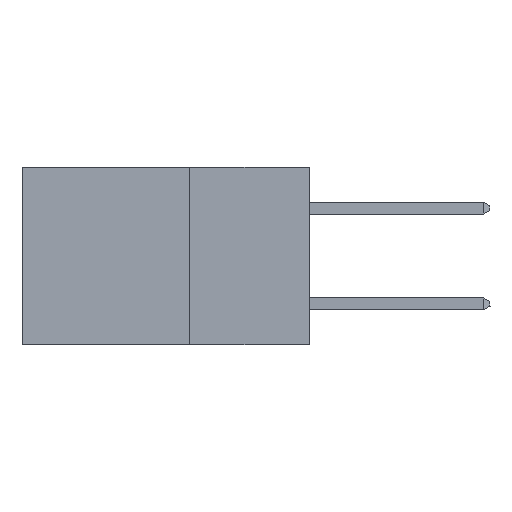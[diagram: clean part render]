
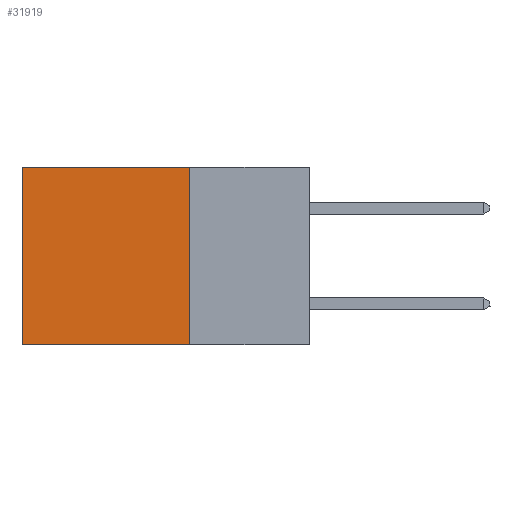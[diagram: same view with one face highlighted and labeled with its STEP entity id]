
A CAD part, left-side view. The second image highlights one B-rep face of the part: STEP entity #31919.
In plain terms, the highlighted planar face has unit normal (-1, 0, 0).
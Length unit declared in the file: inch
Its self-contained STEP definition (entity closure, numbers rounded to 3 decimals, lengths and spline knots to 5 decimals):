
#1154 = VERTEX_POINT ( 'NONE', #10746 ) ;
#1230 = FACE_OUTER_BOUND ( 'NONE', #19401, .T. ) ;
#2661 = PLANE ( 'NONE',  #15347 ) ;
#3942 = DIRECTION ( 'NONE',  ( 0., 0., -1. ) ) ;
#3960 = CARTESIAN_POINT ( 'NONE',  ( 0.2875, 0.25, 0. ) ) ;
#4071 = DIRECTION ( 'NONE',  ( 0., 1., 0. ) ) ;
#8696 = LINE ( 'NONE', #26213, #24119 ) ;
#9492 = CARTESIAN_POINT ( 'NONE',  ( 0.2875, 0.25, 0. ) ) ;
#10141 = LINE ( 'NONE', #36567, #35401 ) ;
#10746 = CARTESIAN_POINT ( 'NONE',  ( 0.2875, 0.6, -0.37 ) ) ;
#11439 = ORIENTED_EDGE ( 'NONE', *, *, #34961, .F. ) ;
#13147 = ORIENTED_EDGE ( 'NONE', *, *, #40397, .T. ) ;
#14121 = CARTESIAN_POINT ( 'NONE',  ( 0.2875, 0.25, 0. ) ) ;
#15347 = AXIS2_PLACEMENT_3D ( 'NONE', #15627, #35400, #35676 ) ;
#15627 = CARTESIAN_POINT ( 'NONE',  ( 0.2875, 0.25, 0. ) ) ;
#15659 = CARTESIAN_POINT ( 'NONE',  ( 0.2875, 0.6, 0. ) ) ;
#16458 = VERTEX_POINT ( 'NONE', #9492 ) ;
#16940 = DIRECTION ( 'NONE',  ( 0., 0., -1. ) ) ;
#19401 = EDGE_LOOP ( 'NONE', ( #13147, #11439, #37066, #22857 ) ) ;
#22857 = ORIENTED_EDGE ( 'NONE', *, *, #39607, .T. ) ;
#23517 = DIRECTION ( 'NONE',  ( 0., 1., 0. ) ) ;
#23641 = VERTEX_POINT ( 'NONE', #36961 ) ;
#24119 = VECTOR ( 'NONE', #4071, 39.37008 ) ;
#25330 = VECTOR ( 'NONE', #3942, 39.37008 ) ;
#26213 = CARTESIAN_POINT ( 'NONE',  ( 0.2875, 0.25, -0.37 ) ) ;
#27415 = LINE ( 'NONE', #14121, #25330 ) ;
#27942 = EDGE_CURVE ( 'NONE', #16458, #23641, #27415, .T. ) ;
#31919 = ADVANCED_FACE ( 'NONE', ( #1230 ), #2661, .F. ) ;
#34961 = EDGE_CURVE ( 'NONE', #23641, #1154, #8696, .T. ) ;
#35400 = DIRECTION ( 'NONE',  ( 1., 0., 0. ) ) ;
#35401 = VECTOR ( 'NONE', #16940, 39.37008 ) ;
#35676 = DIRECTION ( 'NONE',  ( 0., 0., -1. ) ) ;
#36567 = CARTESIAN_POINT ( 'NONE',  ( 0.2875, 0.6, 0. ) ) ;
#36961 = CARTESIAN_POINT ( 'NONE',  ( 0.2875, 0.25, -0.37 ) ) ;
#37043 = VECTOR ( 'NONE', #23517, 39.37008 ) ;
#37066 = ORIENTED_EDGE ( 'NONE', *, *, #27942, .F. ) ;
#39607 = EDGE_CURVE ( 'NONE', #16458, #41908, #41205, .T. ) ;
#40397 = EDGE_CURVE ( 'NONE', #41908, #1154, #10141, .T. ) ;
#41205 = LINE ( 'NONE', #3960, #37043 ) ;
#41908 = VERTEX_POINT ( 'NONE', #15659 ) ;
